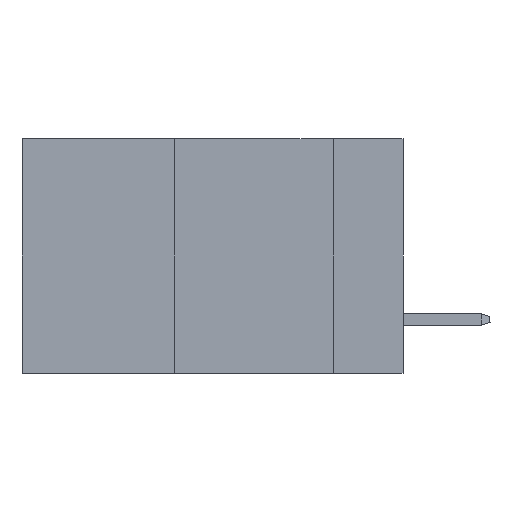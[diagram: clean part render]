
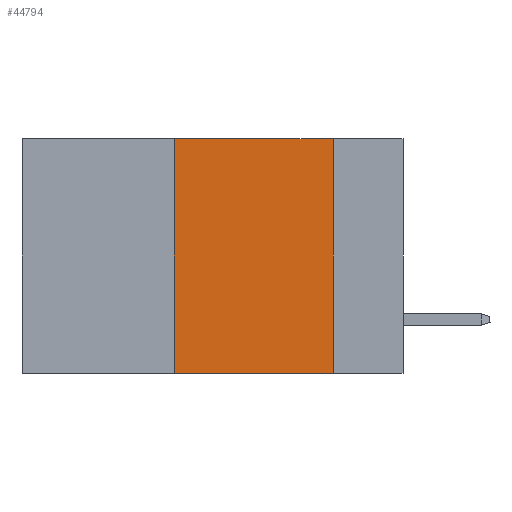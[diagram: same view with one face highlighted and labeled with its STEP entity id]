
A CAD part, left-side view. The second image highlights one B-rep face of the part: STEP entity #44794.
In plain terms, the highlighted planar face has unit normal (-1, 0, 0).
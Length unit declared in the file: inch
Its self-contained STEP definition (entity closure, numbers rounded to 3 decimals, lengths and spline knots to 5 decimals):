
#3096 = CARTESIAN_POINT ( 'NONE',  ( 0., 0.11, -0.37 ) ) ;
#4082 = EDGE_CURVE ( 'NONE', #6140, #27674, #9245, .T. ) ;
#6140 = VERTEX_POINT ( 'NONE', #41725 ) ;
#8830 = VECTOR ( 'NONE', #9976, 39.37008 ) ;
#9245 = LINE ( 'NONE', #35209, #8830 ) ;
#9976 = DIRECTION ( 'NONE',  ( 0., -1., 0. ) ) ;
#11363 = EDGE_LOOP ( 'NONE', ( #20090, #19838, #29952, #18183 ) ) ;
#12188 = VERTEX_POINT ( 'NONE', #38498 ) ;
#14476 = CARTESIAN_POINT ( 'NONE',  ( 0., 0.6, 0. ) ) ;
#15218 = EDGE_CURVE ( 'NONE', #37021, #27674, #27846, .T. ) ;
#16269 = LINE ( 'NONE', #27031, #35426 ) ;
#17186 = PLANE ( 'NONE',  #20522 ) ;
#18183 = ORIENTED_EDGE ( 'NONE', *, *, #4082, .T. ) ;
#18232 = DIRECTION ( 'NONE',  ( 0., -1., 0. ) ) ;
#18744 = CARTESIAN_POINT ( 'NONE',  ( 0., 0.11, 0. ) ) ;
#18948 = CARTESIAN_POINT ( 'NONE',  ( 0., 0.6, 0. ) ) ;
#19838 = ORIENTED_EDGE ( 'NONE', *, *, #30830, .F. ) ;
#20090 = ORIENTED_EDGE ( 'NONE', *, *, #15218, .F. ) ;
#20299 = EDGE_CURVE ( 'NONE', #6140, #12188, #16269, .T. ) ;
#20522 = AXIS2_PLACEMENT_3D ( 'NONE', #14476, #47264, #35764 ) ;
#23681 = CARTESIAN_POINT ( 'NONE',  ( 0., 0.11, 0. ) ) ;
#27031 = CARTESIAN_POINT ( 'NONE',  ( 0., 0.36, 0. ) ) ;
#27477 = VECTOR ( 'NONE', #38615, 39.37008 ) ;
#27674 = VERTEX_POINT ( 'NONE', #3096 ) ;
#27846 = LINE ( 'NONE', #23681, #27477 ) ;
#29952 = ORIENTED_EDGE ( 'NONE', *, *, #20299, .F. ) ;
#30830 = EDGE_CURVE ( 'NONE', #12188, #37021, #36826, .T. ) ;
#35209 = CARTESIAN_POINT ( 'NONE',  ( 0., 0.6, -0.37 ) ) ;
#35426 = VECTOR ( 'NONE', #41947, 39.37008 ) ;
#35764 = DIRECTION ( 'NONE',  ( 0., 0., -1. ) ) ;
#36826 = LINE ( 'NONE', #18948, #43911 ) ;
#37021 = VERTEX_POINT ( 'NONE', #18744 ) ;
#38498 = CARTESIAN_POINT ( 'NONE',  ( 0., 0.36, 0. ) ) ;
#38615 = DIRECTION ( 'NONE',  ( 0., 0., -1. ) ) ;
#41725 = CARTESIAN_POINT ( 'NONE',  ( 0., 0.36, -0.37 ) ) ;
#41947 = DIRECTION ( 'NONE',  ( 0., 0., 1. ) ) ;
#43125 = FACE_OUTER_BOUND ( 'NONE', #11363, .T. ) ;
#43911 = VECTOR ( 'NONE', #18232, 39.37008 ) ;
#44794 = ADVANCED_FACE ( 'NONE', ( #43125 ), #17186, .F. ) ;
#47264 = DIRECTION ( 'NONE',  ( 1., 0., 0. ) ) ;
